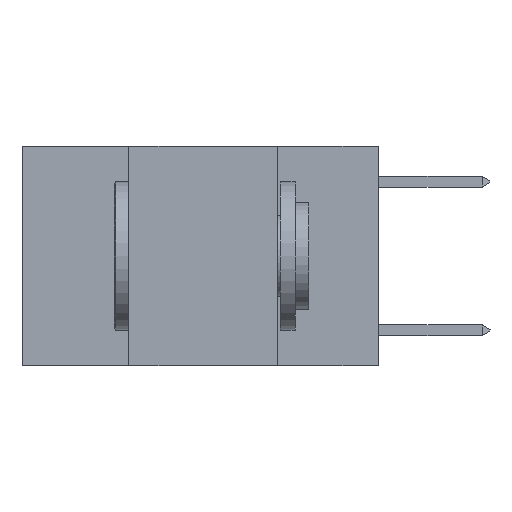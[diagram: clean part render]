
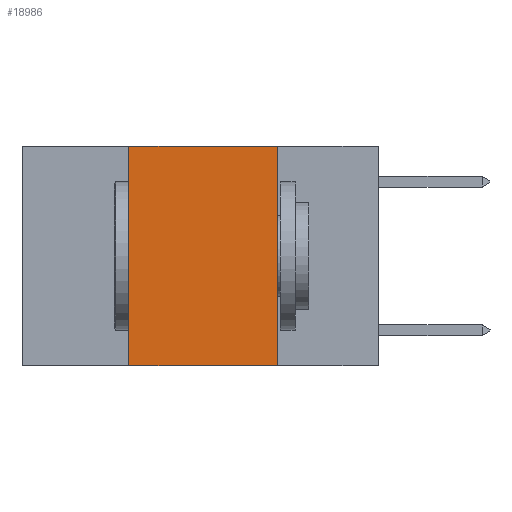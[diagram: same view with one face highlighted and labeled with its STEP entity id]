
A CAD part, left-side view. The second image highlights one B-rep face of the part: STEP entity #18986.
In plain terms, the highlighted planar face has unit normal (-1, 0, 0).
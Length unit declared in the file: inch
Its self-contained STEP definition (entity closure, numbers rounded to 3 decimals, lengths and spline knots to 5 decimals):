
#167 = CARTESIAN_POINT ( 'NONE',  ( 0., 0.42, -0.37 ) ) ;
#713 = DIRECTION ( 'NONE',  ( 0., 0., -1. ) ) ;
#2147 = EDGE_LOOP ( 'NONE', ( #7118, #7191, #7528, #9078 ) ) ;
#2161 = LINE ( 'NONE', #11055, #8002 ) ;
#3805 = DIRECTION ( 'NONE',  ( 0., -1., 0. ) ) ;
#3825 = CARTESIAN_POINT ( 'NONE',  ( 0., 0.17, 0. ) ) ;
#7118 = ORIENTED_EDGE ( 'NONE', *, *, #24236, .F. ) ;
#7191 = ORIENTED_EDGE ( 'NONE', *, *, #22462, .F. ) ;
#7352 = DIRECTION ( 'NONE',  ( 0., 0., 1. ) ) ;
#7528 = ORIENTED_EDGE ( 'NONE', *, *, #18754, .F. ) ;
#8002 = VECTOR ( 'NONE', #30345, 39.37008 ) ;
#9078 = ORIENTED_EDGE ( 'NONE', *, *, #23649, .T. ) ;
#9776 = CARTESIAN_POINT ( 'NONE',  ( 0., 0.42, 0. ) ) ;
#9867 = CARTESIAN_POINT ( 'NONE',  ( 0., 0.17, -0.37 ) ) ;
#10267 = CARTESIAN_POINT ( 'NONE',  ( 0., 0.42, 0. ) ) ;
#10499 = CARTESIAN_POINT ( 'NONE',  ( 0., 0.6, 0. ) ) ;
#10982 = DIRECTION ( 'NONE',  ( 0., -1., 0. ) ) ;
#11055 = CARTESIAN_POINT ( 'NONE',  ( 0., 0.17, 0. ) ) ;
#11080 = LINE ( 'NONE', #18331, #29559 ) ;
#14595 = VERTEX_POINT ( 'NONE', #9867 ) ;
#15297 = DIRECTION ( 'NONE',  ( 1., 0., 0. ) ) ;
#15666 = CARTESIAN_POINT ( 'NONE',  ( 0., 0.6, 0. ) ) ;
#16933 = VECTOR ( 'NONE', #7352, 39.37008 ) ;
#17882 = VERTEX_POINT ( 'NONE', #3825 ) ;
#17889 = VECTOR ( 'NONE', #10982, 39.37008 ) ;
#18331 = CARTESIAN_POINT ( 'NONE',  ( 0., 0.6, -0.37 ) ) ;
#18474 = LINE ( 'NONE', #9776, #16933 ) ;
#18666 = LINE ( 'NONE', #15666, #17889 ) ;
#18754 = EDGE_CURVE ( 'NONE', #25924, #24699, #18474, .T. ) ;
#18986 = ADVANCED_FACE ( 'NONE', ( #30611 ), #22530, .F. ) ;
#22462 = EDGE_CURVE ( 'NONE', #24699, #17882, #18666, .T. ) ;
#22530 = PLANE ( 'NONE',  #30487 ) ;
#23649 = EDGE_CURVE ( 'NONE', #25924, #14595, #11080, .T. ) ;
#24236 = EDGE_CURVE ( 'NONE', #17882, #14595, #2161, .T. ) ;
#24699 = VERTEX_POINT ( 'NONE', #10267 ) ;
#25924 = VERTEX_POINT ( 'NONE', #167 ) ;
#29559 = VECTOR ( 'NONE', #3805, 39.37008 ) ;
#30345 = DIRECTION ( 'NONE',  ( 0., 0., -1. ) ) ;
#30487 = AXIS2_PLACEMENT_3D ( 'NONE', #10499, #15297, #713 ) ;
#30611 = FACE_OUTER_BOUND ( 'NONE', #2147, .T. ) ;
